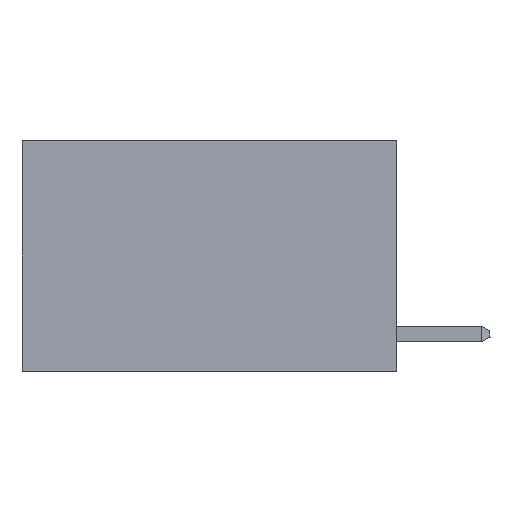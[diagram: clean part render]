
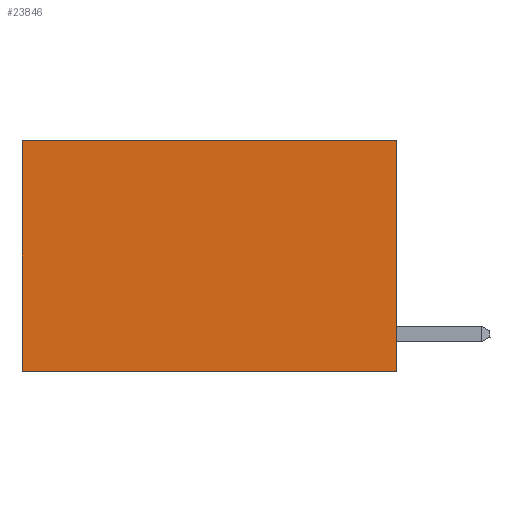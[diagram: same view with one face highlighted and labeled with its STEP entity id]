
A CAD part, left-side view. The second image highlights one B-rep face of the part: STEP entity #23846.
In plain terms, the highlighted planar face has unit normal (-1, 0, 0).
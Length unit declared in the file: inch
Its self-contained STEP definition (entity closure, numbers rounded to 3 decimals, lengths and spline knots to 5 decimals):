
#203 = FACE_OUTER_BOUND ( 'NONE', #764, .T. ) ;
#334 = DIRECTION ( 'NONE',  ( 1., 0., 0. ) ) ;
#456 = DIRECTION ( 'NONE',  ( 0., 0., -1. ) ) ;
#587 = VECTOR ( 'NONE', #1703, 39.37008 ) ;
#744 = VERTEX_POINT ( 'NONE', #22963 ) ;
#764 = EDGE_LOOP ( 'NONE', ( #20821, #18279, #7214, #25292 ) ) ;
#1703 = DIRECTION ( 'NONE',  ( 0., 0., -1. ) ) ;
#1734 = VECTOR ( 'NONE', #9394, 39.37008 ) ;
#2258 = EDGE_CURVE ( 'NONE', #24806, #16448, #19158, .T. ) ;
#2884 = VECTOR ( 'NONE', #23235, 39.37008 ) ;
#3167 = VECTOR ( 'NONE', #18918, 39.37008 ) ;
#3415 = CARTESIAN_POINT ( 'NONE',  ( 0.2625, 0., -0.37 ) ) ;
#3660 = CARTESIAN_POINT ( 'NONE',  ( 0.2625, 0.6, -0.37 ) ) ;
#4292 = EDGE_CURVE ( 'NONE', #9703, #16448, #20709, .T. ) ;
#6317 = PLANE ( 'NONE',  #14050 ) ;
#7214 = ORIENTED_EDGE ( 'NONE', *, *, #24153, .F. ) ;
#9394 = DIRECTION ( 'NONE',  ( 0., 0., -1. ) ) ;
#9473 = LINE ( 'NONE', #19370, #2884 ) ;
#9703 = VERTEX_POINT ( 'NONE', #3415 ) ;
#10042 = CARTESIAN_POINT ( 'NONE',  ( 0.2625, 0., 0. ) ) ;
#14050 = AXIS2_PLACEMENT_3D ( 'NONE', #10042, #334, #456 ) ;
#16448 = VERTEX_POINT ( 'NONE', #3660 ) ;
#17682 = EDGE_CURVE ( 'NONE', #744, #24806, #9473, .T. ) ;
#18279 = ORIENTED_EDGE ( 'NONE', *, *, #4292, .F. ) ;
#18918 = DIRECTION ( 'NONE',  ( 0., 1., 0. ) ) ;
#19158 = LINE ( 'NONE', #23283, #1734 ) ;
#19176 = CARTESIAN_POINT ( 'NONE',  ( 0.2625, 0., -0.37 ) ) ;
#19370 = CARTESIAN_POINT ( 'NONE',  ( 0.2625, 0., 0. ) ) ;
#20709 = LINE ( 'NONE', #19176, #3167 ) ;
#20821 = ORIENTED_EDGE ( 'NONE', *, *, #2258, .T. ) ;
#21007 = LINE ( 'NONE', #21141, #587 ) ;
#21141 = CARTESIAN_POINT ( 'NONE',  ( 0.2625, 0., 0. ) ) ;
#21630 = CARTESIAN_POINT ( 'NONE',  ( 0.2625, 0.6, 0. ) ) ;
#22963 = CARTESIAN_POINT ( 'NONE',  ( 0.2625, 0., 0. ) ) ;
#23235 = DIRECTION ( 'NONE',  ( 0., 1., 0. ) ) ;
#23283 = CARTESIAN_POINT ( 'NONE',  ( 0.2625, 0.6, 0. ) ) ;
#23846 = ADVANCED_FACE ( 'NONE', ( #203 ), #6317, .F. ) ;
#24153 = EDGE_CURVE ( 'NONE', #744, #9703, #21007, .T. ) ;
#24806 = VERTEX_POINT ( 'NONE', #21630 ) ;
#25292 = ORIENTED_EDGE ( 'NONE', *, *, #17682, .T. ) ;
